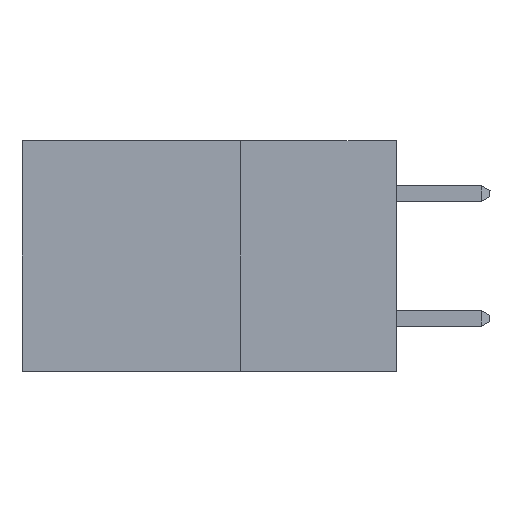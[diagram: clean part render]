
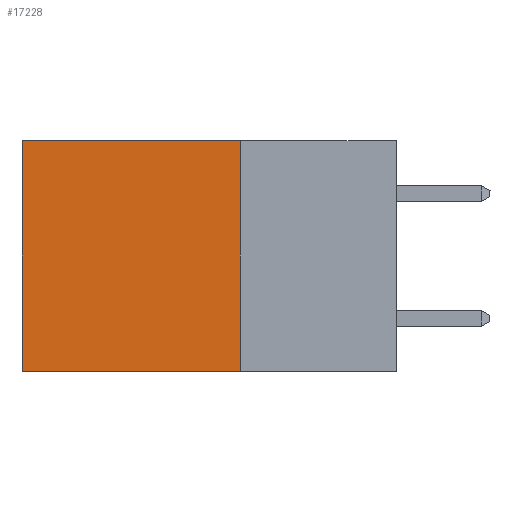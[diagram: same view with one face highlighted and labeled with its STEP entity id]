
A CAD part, left-side view. The second image highlights one B-rep face of the part: STEP entity #17228.
In plain terms, the highlighted planar face has unit normal (-1, 0, 0).
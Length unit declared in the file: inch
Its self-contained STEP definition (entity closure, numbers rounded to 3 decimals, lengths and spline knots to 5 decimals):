
#1085 = VECTOR ( 'NONE', #8468, 39.37008 ) ;
#1201 = VECTOR ( 'NONE', #16593, 39.37008 ) ;
#1343 = CARTESIAN_POINT ( 'NONE',  ( 0.298, 0.6, 0. ) ) ;
#1344 = ORIENTED_EDGE ( 'NONE', *, *, #8170, .F. ) ;
#3180 = DIRECTION ( 'NONE',  ( 0., 0., -1. ) ) ;
#4208 = EDGE_CURVE ( 'NONE', #4459, #5271, #17318, .T. ) ;
#4459 = VERTEX_POINT ( 'NONE', #7980 ) ;
#5271 = VERTEX_POINT ( 'NONE', #12938 ) ;
#5427 = LINE ( 'NONE', #1343, #1201 ) ;
#5570 = AXIS2_PLACEMENT_3D ( 'NONE', #8939, #16383, #11953 ) ;
#5988 = ORIENTED_EDGE ( 'NONE', *, *, #18107, .F. ) ;
#6286 = ORIENTED_EDGE ( 'NONE', *, *, #10413, .T. ) ;
#6991 = LINE ( 'NONE', #12320, #14958 ) ;
#7980 = CARTESIAN_POINT ( 'NONE',  ( 0.298, 0.25, 0. ) ) ;
#8170 = EDGE_CURVE ( 'NONE', #13840, #18222, #17959, .T. ) ;
#8468 = DIRECTION ( 'NONE',  ( 0., 1., 0. ) ) ;
#8538 = CARTESIAN_POINT ( 'NONE',  ( 0.298, 0.25, 0. ) ) ;
#8939 = CARTESIAN_POINT ( 'NONE',  ( 0.298, 0.25, 0. ) ) ;
#9304 = DIRECTION ( 'NONE',  ( 0., 1., 0. ) ) ;
#9517 = VECTOR ( 'NONE', #9304, 39.37008 ) ;
#9544 = CARTESIAN_POINT ( 'NONE',  ( 0.298, 0.6, -0.37 ) ) ;
#10410 = PLANE ( 'NONE',  #5570 ) ;
#10413 = EDGE_CURVE ( 'NONE', #5271, #18222, #5427, .T. ) ;
#11214 = CARTESIAN_POINT ( 'NONE',  ( 0.298, 0.25, -0.37 ) ) ;
#11953 = DIRECTION ( 'NONE',  ( 0., 0., -1. ) ) ;
#12320 = CARTESIAN_POINT ( 'NONE',  ( 0.298, 0.25, 0. ) ) ;
#12938 = CARTESIAN_POINT ( 'NONE',  ( 0.298, 0.6, 0. ) ) ;
#13840 = VERTEX_POINT ( 'NONE', #15525 ) ;
#14958 = VECTOR ( 'NONE', #3180, 39.37008 ) ;
#15525 = CARTESIAN_POINT ( 'NONE',  ( 0.298, 0.25, -0.37 ) ) ;
#16383 = DIRECTION ( 'NONE',  ( 1., 0., 0. ) ) ;
#16593 = DIRECTION ( 'NONE',  ( 0., 0., -1. ) ) ;
#17228 = ADVANCED_FACE ( 'NONE', ( #19426 ), #10410, .F. ) ;
#17318 = LINE ( 'NONE', #8538, #1085 ) ;
#17959 = LINE ( 'NONE', #11214, #9517 ) ;
#18053 = ORIENTED_EDGE ( 'NONE', *, *, #4208, .T. ) ;
#18107 = EDGE_CURVE ( 'NONE', #4459, #13840, #6991, .T. ) ;
#18222 = VERTEX_POINT ( 'NONE', #9544 ) ;
#19277 = EDGE_LOOP ( 'NONE', ( #6286, #1344, #5988, #18053 ) ) ;
#19426 = FACE_OUTER_BOUND ( 'NONE', #19277, .T. ) ;
